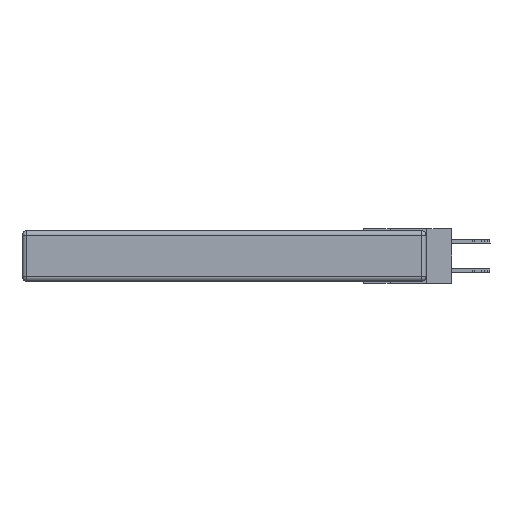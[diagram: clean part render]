
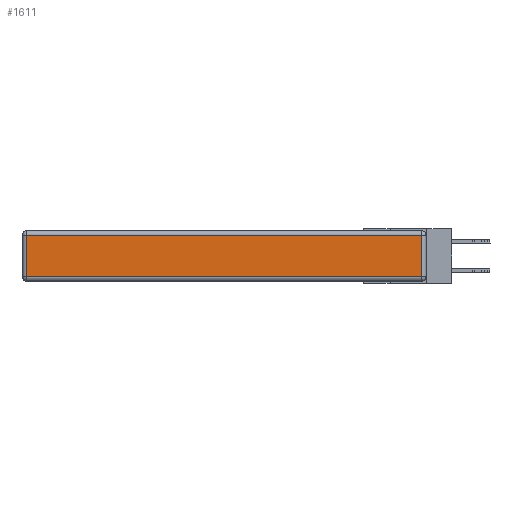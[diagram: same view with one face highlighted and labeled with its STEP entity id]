
A CAD part, left-side view. The second image highlights one B-rep face of the part: STEP entity #1611.
In plain terms, the highlighted planar face has unit normal (-1, 0, 0).
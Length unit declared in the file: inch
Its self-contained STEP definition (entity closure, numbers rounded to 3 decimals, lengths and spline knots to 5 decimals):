
#1611 = ADVANCED_FACE ( 'NONE', ( #23116 ), #8496, .T. ) ;
#2368 = VERTEX_POINT ( 'NONE', #13205 ) ;
#3637 = EDGE_LOOP ( 'NONE', ( #5351, #13398, #24880, #15453 ) ) ;
#4560 = LINE ( 'NONE', #13604, #7686 ) ;
#5351 = ORIENTED_EDGE ( 'NONE', *, *, #20058, .T. ) ;
#6900 = VERTEX_POINT ( 'NONE', #17523 ) ;
#6946 = EDGE_CURVE ( 'NONE', #6900, #14505, #4560, .T. ) ;
#7686 = VECTOR ( 'NONE', #31277, 39.37008 ) ;
#8496 = PLANE ( 'NONE',  #16954 ) ;
#8746 = CARTESIAN_POINT ( 'NONE',  ( 0., 0.03, -0.03 ) ) ;
#8911 = CARTESIAN_POINT ( 'NONE',  ( 0., 2.72, -0.313 ) ) ;
#10567 = VERTEX_POINT ( 'NONE', #8746 ) ;
#10884 = DIRECTION ( 'NONE',  ( -1., 0., 0. ) ) ;
#11105 = CARTESIAN_POINT ( 'NONE',  ( 0., 0.03, -0.343 ) ) ;
#13205 = CARTESIAN_POINT ( 'NONE',  ( 0., 0.03, -0.313 ) ) ;
#13398 = ORIENTED_EDGE ( 'NONE', *, *, #27983, .T. ) ;
#13604 = CARTESIAN_POINT ( 'NONE',  ( 0., 2.72, -0.343 ) ) ;
#14505 = VERTEX_POINT ( 'NONE', #8911 ) ;
#15453 = ORIENTED_EDGE ( 'NONE', *, *, #6946, .T. ) ;
#16914 = CARTESIAN_POINT ( 'NONE',  ( 0., 2.75, -0.03 ) ) ;
#16954 = AXIS2_PLACEMENT_3D ( 'NONE', #25771, #10884, #30729 ) ;
#17523 = CARTESIAN_POINT ( 'NONE',  ( 0., 2.72, -0.03 ) ) ;
#20058 = EDGE_CURVE ( 'NONE', #14505, #2368, #27044, .T. ) ;
#21179 = LINE ( 'NONE', #11105, #28903 ) ;
#22596 = LINE ( 'NONE', #16914, #26877 ) ;
#23116 = FACE_OUTER_BOUND ( 'NONE', #3637, .T. ) ;
#23510 = DIRECTION ( 'NONE',  ( 0., 0., 1. ) ) ;
#24591 = EDGE_CURVE ( 'NONE', #10567, #6900, #22596, .T. ) ;
#24880 = ORIENTED_EDGE ( 'NONE', *, *, #24591, .T. ) ;
#25449 = VECTOR ( 'NONE', #26158, 39.37008 ) ;
#25771 = CARTESIAN_POINT ( 'NONE',  ( 0., 0., -0.343 ) ) ;
#26158 = DIRECTION ( 'NONE',  ( 0., -1., 0. ) ) ;
#26877 = VECTOR ( 'NONE', #26932, 39.37008 ) ;
#26932 = DIRECTION ( 'NONE',  ( 0., 1., 0. ) ) ;
#27044 = LINE ( 'NONE', #29268, #25449 ) ;
#27983 = EDGE_CURVE ( 'NONE', #2368, #10567, #21179, .T. ) ;
#28903 = VECTOR ( 'NONE', #23510, 39.37008 ) ;
#29268 = CARTESIAN_POINT ( 'NONE',  ( 0., 0., -0.313 ) ) ;
#30729 = DIRECTION ( 'NONE',  ( 0., 0., 1. ) ) ;
#31277 = DIRECTION ( 'NONE',  ( 0., 0., -1. ) ) ;
